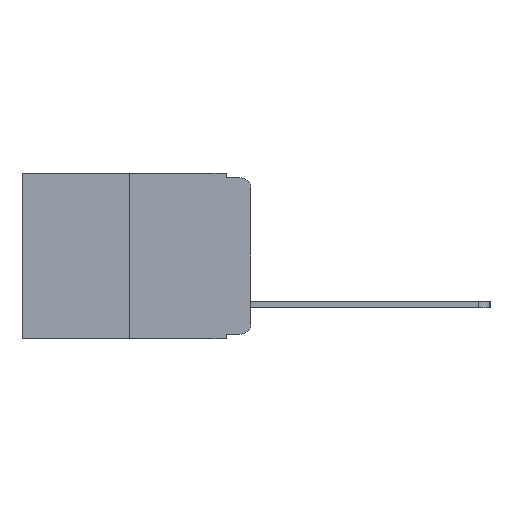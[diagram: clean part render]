
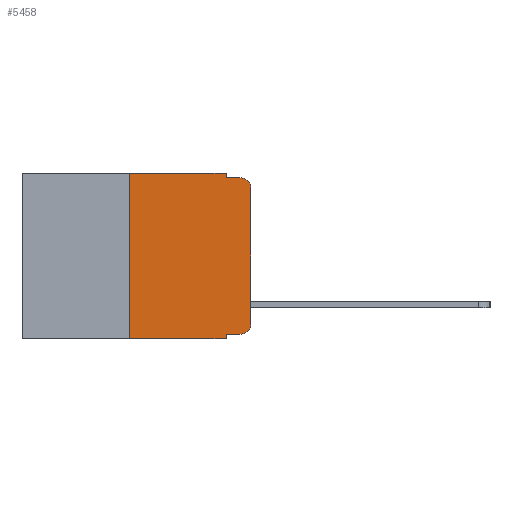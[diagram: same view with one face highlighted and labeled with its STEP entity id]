
A CAD part, left-side view. The second image highlights one B-rep face of the part: STEP entity #5458.
In plain terms, the highlighted planar face has unit normal (-1, 0, 0).
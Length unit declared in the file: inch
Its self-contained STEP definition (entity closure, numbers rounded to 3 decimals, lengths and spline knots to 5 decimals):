
#8 = ORIENTED_EDGE ( 'NONE', *, *, #6768, .T. ) ;
#28 = CARTESIAN_POINT ( 'NONE',  ( 0., 0.25, 0. ) ) ;
#161 = EDGE_CURVE ( 'NONE', #2118, #304, #14486, .T. ) ;
#283 = ORIENTED_EDGE ( 'NONE', *, *, #6470, .T. ) ;
#304 = VERTEX_POINT ( 'NONE', #14151 ) ;
#335 = CARTESIAN_POINT ( 'NONE',  ( 0., 0.473, -0.343 ) ) ;
#715 = DIRECTION ( 'NONE',  ( 0., 0., -1. ) ) ;
#833 = CARTESIAN_POINT ( 'NONE',  ( 0., 0., -0.313 ) ) ;
#1320 = ORIENTED_EDGE ( 'NONE', *, *, #5141, .T. ) ;
#1405 = VERTEX_POINT ( 'NONE', #1955 ) ;
#1521 = LINE ( 'NONE', #5382, #4509 ) ;
#1723 = DIRECTION ( 'NONE',  ( 0., -1., 0. ) ) ;
#1736 = EDGE_LOOP ( 'NONE', ( #5342, #283, #8264, #7246, #13276, #5079, #5863, #5469, #8, #1320 ) ) ;
#1883 = VERTEX_POINT ( 'NONE', #14945 ) ;
#1955 = CARTESIAN_POINT ( 'NONE',  ( 0., 0.02, -0.333 ) ) ;
#1993 = CARTESIAN_POINT ( 'NONE',  ( 0., 0.051, -0.01 ) ) ;
#2031 = CIRCLE ( 'NONE', #10503, 0.02 ) ;
#2118 = VERTEX_POINT ( 'NONE', #28 ) ;
#2520 = DIRECTION ( 'NONE',  ( 0., 0., 1. ) ) ;
#3096 = CARTESIAN_POINT ( 'NONE',  ( 0., 0.25, 0. ) ) ;
#3110 = VECTOR ( 'NONE', #4346, 39.37008 ) ;
#3599 = VERTEX_POINT ( 'NONE', #833 ) ;
#3782 = DIRECTION ( 'NONE',  ( -1., 0., 0. ) ) ;
#3980 = EDGE_CURVE ( 'NONE', #6443, #1883, #8635, .T. ) ;
#4346 = DIRECTION ( 'NONE',  ( 0., 0., 1. ) ) ;
#4509 = VECTOR ( 'NONE', #6598, 39.37008 ) ;
#4757 = VERTEX_POINT ( 'NONE', #11868 ) ;
#5079 = ORIENTED_EDGE ( 'NONE', *, *, #9036, .F. ) ;
#5141 = EDGE_CURVE ( 'NONE', #1405, #3599, #2031, .T. ) ;
#5342 = ORIENTED_EDGE ( 'NONE', *, *, #9486, .T. ) ;
#5382 = CARTESIAN_POINT ( 'NONE',  ( 0., 0.051, 0. ) ) ;
#5458 = ADVANCED_FACE ( 'NONE', ( #6515 ), #13583, .F. ) ;
#5469 = ORIENTED_EDGE ( 'NONE', *, *, #7549, .F. ) ;
#5863 = ORIENTED_EDGE ( 'NONE', *, *, #11604, .T. ) ;
#5989 = CARTESIAN_POINT ( 'NONE',  ( 0., 0.051, -0.01 ) ) ;
#5997 = CARTESIAN_POINT ( 'NONE',  ( 0., 0.051, -0.333 ) ) ;
#6001 = CARTESIAN_POINT ( 'NONE',  ( 0., 0., -0.03 ) ) ;
#6310 = CARTESIAN_POINT ( 'NONE',  ( 0., 0.051, -0.333 ) ) ;
#6443 = VERTEX_POINT ( 'NONE', #5989 ) ;
#6470 = EDGE_CURVE ( 'NONE', #6638, #1883, #10501, .T. ) ;
#6515 = FACE_OUTER_BOUND ( 'NONE', #1736, .T. ) ;
#6598 = DIRECTION ( 'NONE',  ( 0., 0., -1. ) ) ;
#6638 = VERTEX_POINT ( 'NONE', #6001 ) ;
#6657 = LINE ( 'NONE', #6310, #11860 ) ;
#6768 = EDGE_CURVE ( 'NONE', #8664, #1405, #6657, .T. ) ;
#6799 = AXIS2_PLACEMENT_3D ( 'NONE', #13820, #7283, #14900 ) ;
#7246 = ORIENTED_EDGE ( 'NONE', *, *, #10495, .F. ) ;
#7283 = DIRECTION ( 'NONE',  ( -1., 0., 0. ) ) ;
#7549 = EDGE_CURVE ( 'NONE', #8664, #12645, #1521, .T. ) ;
#8147 = DIRECTION ( 'NONE',  ( 1., 0., 0. ) ) ;
#8264 = ORIENTED_EDGE ( 'NONE', *, *, #3980, .F. ) ;
#8512 = DIRECTION ( 'NONE',  ( 0., 0., -1. ) ) ;
#8635 = LINE ( 'NONE', #1993, #9663 ) ;
#8664 = VERTEX_POINT ( 'NONE', #5997 ) ;
#9036 = EDGE_CURVE ( 'NONE', #4757, #2118, #9412, .T. ) ;
#9412 = LINE ( 'NONE', #3096, #3110 ) ;
#9486 = EDGE_CURVE ( 'NONE', #3599, #6638, #9740, .T. ) ;
#9663 = VECTOR ( 'NONE', #10293, 39.37008 ) ;
#9740 = LINE ( 'NONE', #10795, #14815 ) ;
#10011 = VECTOR ( 'NONE', #1723, 39.37008 ) ;
#10293 = DIRECTION ( 'NONE',  ( 0., -1., 0. ) ) ;
#10495 = EDGE_CURVE ( 'NONE', #304, #6443, #11421, .T. ) ;
#10501 = CIRCLE ( 'NONE', #6799, 0.02 ) ;
#10503 = AXIS2_PLACEMENT_3D ( 'NONE', #10746, #3782, #11850 ) ;
#10684 = AXIS2_PLACEMENT_3D ( 'NONE', #14647, #8147, #715 ) ;
#10746 = CARTESIAN_POINT ( 'NONE',  ( 0., 0.02, -0.313 ) ) ;
#10795 = CARTESIAN_POINT ( 'NONE',  ( 0., 0., 0. ) ) ;
#11421 = LINE ( 'NONE', #11762, #13951 ) ;
#11604 = EDGE_CURVE ( 'NONE', #4757, #12645, #12588, .T. ) ;
#11762 = CARTESIAN_POINT ( 'NONE',  ( 0., 0.051, 0. ) ) ;
#11843 = CARTESIAN_POINT ( 'NONE',  ( 0., 0.473, 0. ) ) ;
#11850 = DIRECTION ( 'NONE',  ( 0., 0., -1. ) ) ;
#11860 = VECTOR ( 'NONE', #11864, 39.37008 ) ;
#11864 = DIRECTION ( 'NONE',  ( 0., -1., 0. ) ) ;
#11868 = CARTESIAN_POINT ( 'NONE',  ( 0., 0.25, -0.343 ) ) ;
#11919 = DIRECTION ( 'NONE',  ( 0., -1., 0. ) ) ;
#12588 = LINE ( 'NONE', #335, #10011 ) ;
#12645 = VERTEX_POINT ( 'NONE', #13056 ) ;
#13056 = CARTESIAN_POINT ( 'NONE',  ( 0., 0.051, -0.343 ) ) ;
#13276 = ORIENTED_EDGE ( 'NONE', *, *, #161, .F. ) ;
#13583 = PLANE ( 'NONE',  #10684 ) ;
#13820 = CARTESIAN_POINT ( 'NONE',  ( 0., 0.02, -0.03 ) ) ;
#13951 = VECTOR ( 'NONE', #8512, 39.37008 ) ;
#14151 = CARTESIAN_POINT ( 'NONE',  ( 0., 0.051, 0. ) ) ;
#14167 = VECTOR ( 'NONE', #11919, 39.37008 ) ;
#14486 = LINE ( 'NONE', #11843, #14167 ) ;
#14647 = CARTESIAN_POINT ( 'NONE',  ( 0., 0.473, 0. ) ) ;
#14815 = VECTOR ( 'NONE', #2520, 39.37008 ) ;
#14900 = DIRECTION ( 'NONE',  ( 0., 0., -1. ) ) ;
#14945 = CARTESIAN_POINT ( 'NONE',  ( 0., 0.02, -0.01 ) ) ;
